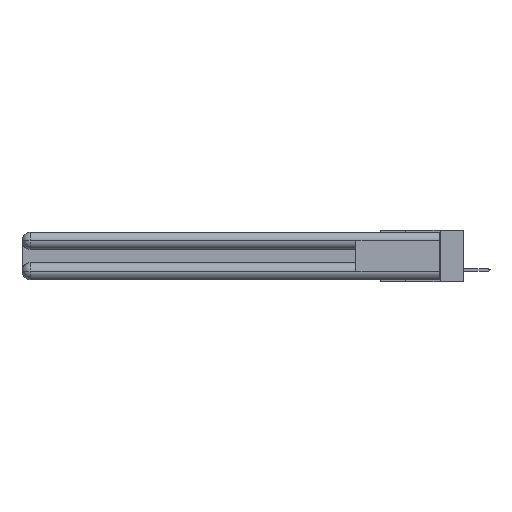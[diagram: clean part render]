
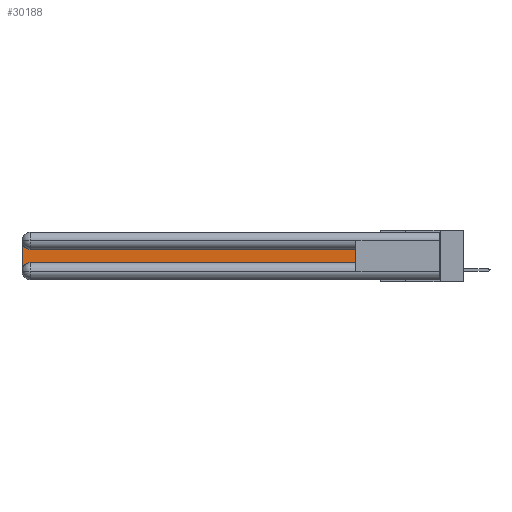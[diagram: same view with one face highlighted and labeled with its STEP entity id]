
A CAD part, left-side view. The second image highlights one B-rep face of the part: STEP entity #30188.
In plain terms, the highlighted planar face has unit normal (-1, 0, 0).
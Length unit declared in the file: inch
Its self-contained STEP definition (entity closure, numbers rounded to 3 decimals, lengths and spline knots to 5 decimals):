
#1519 = CIRCLE ( 'NONE', #22142, 0.06 ) ;
#1719 = CARTESIAN_POINT ( 'NONE',  ( 0.075, 3., -0.2175 ) ) ;
#1810 = LINE ( 'NONE', #1719, #28966 ) ;
#3148 = AXIS2_PLACEMENT_3D ( 'NONE', #26967, #32387, #3386 ) ;
#3265 = AXIS2_PLACEMENT_3D ( 'NONE', #26325, #26096, #31637 ) ;
#3386 = DIRECTION ( 'NONE',  ( 0., 0., -1. ) ) ;
#3557 = VECTOR ( 'NONE', #33413, 39.37008 ) ;
#4754 = ORIENTED_EDGE ( 'NONE', *, *, #8854, .T. ) ;
#5421 = CARTESIAN_POINT ( 'NONE',  ( 0.075, 0.6, -0.1225 ) ) ;
#5508 = VECTOR ( 'NONE', #16641, 39.37008 ) ;
#5574 = VERTEX_POINT ( 'NONE', #25280 ) ;
#8219 = VERTEX_POINT ( 'NONE', #13846 ) ;
#8854 = EDGE_CURVE ( 'NONE', #5574, #23633, #11387, .T. ) ;
#11274 = LINE ( 'NONE', #16530, #5508 ) ;
#11387 = CIRCLE ( 'NONE', #3148, 0.06 ) ;
#11801 = CARTESIAN_POINT ( 'NONE',  ( 0.075, 3., -0.2775 ) ) ;
#12319 = ORIENTED_EDGE ( 'NONE', *, *, #27634, .T. ) ;
#12581 = VERTEX_POINT ( 'NONE', #11801 ) ;
#13846 = CARTESIAN_POINT ( 'NONE',  ( 0.075, 2.94, -0.2175 ) ) ;
#13995 = ORIENTED_EDGE ( 'NONE', *, *, #14472, .T. ) ;
#14472 = EDGE_CURVE ( 'NONE', #23633, #12581, #1810, .T. ) ;
#16456 = CARTESIAN_POINT ( 'NONE',  ( 0.075, 2.94, -0.2775 ) ) ;
#16530 = CARTESIAN_POINT ( 'NONE',  ( 0.075, 0.6, -0.2175 ) ) ;
#16641 = DIRECTION ( 'NONE',  ( 0., -1., 0. ) ) ;
#18479 = EDGE_CURVE ( 'NONE', #8219, #20541, #11274, .T. ) ;
#20536 = CARTESIAN_POINT ( 'NONE',  ( 0.075, 0.6, -0.2175 ) ) ;
#20541 = VERTEX_POINT ( 'NONE', #26235 ) ;
#20821 = PLANE ( 'NONE',  #3265 ) ;
#21967 = EDGE_CURVE ( 'NONE', #12581, #8219, #1519, .T. ) ;
#22107 = FACE_OUTER_BOUND ( 'NONE', #31249, .T. ) ;
#22142 = AXIS2_PLACEMENT_3D ( 'NONE', #16456, #26698, #31997 ) ;
#22172 = VECTOR ( 'NONE', #33211, 39.37008 ) ;
#22885 = DIRECTION ( 'NONE',  ( 0., 0., -1. ) ) ;
#23083 = VERTEX_POINT ( 'NONE', #5421 ) ;
#23546 = CARTESIAN_POINT ( 'NONE',  ( 0.075, 3., -0.0625 ) ) ;
#23633 = VERTEX_POINT ( 'NONE', #23546 ) ;
#25280 = CARTESIAN_POINT ( 'NONE',  ( 0.075, 2.94, -0.1225 ) ) ;
#25559 = ORIENTED_EDGE ( 'NONE', *, *, #21967, .T. ) ;
#26096 = DIRECTION ( 'NONE',  ( 1., 0., 0. ) ) ;
#26235 = CARTESIAN_POINT ( 'NONE',  ( 0.075, 0.6, -0.2175 ) ) ;
#26325 = CARTESIAN_POINT ( 'NONE',  ( 0.075, 3., -0.1225 ) ) ;
#26698 = DIRECTION ( 'NONE',  ( 1., 0., 0. ) ) ;
#26967 = CARTESIAN_POINT ( 'NONE',  ( 0.075, 2.94, -0.0625 ) ) ;
#27580 = CARTESIAN_POINT ( 'NONE',  ( 0.075, 0.6, -0.1225 ) ) ;
#27634 = EDGE_CURVE ( 'NONE', #20541, #23083, #28610, .T. ) ;
#28610 = LINE ( 'NONE', #20536, #3557 ) ;
#28713 = LINE ( 'NONE', #27580, #22172 ) ;
#28966 = VECTOR ( 'NONE', #22885, 39.37008 ) ;
#29650 = EDGE_CURVE ( 'NONE', #23083, #5574, #28713, .T. ) ;
#30188 = ADVANCED_FACE ( 'NONE', ( #22107 ), #20821, .F. ) ;
#31249 = EDGE_LOOP ( 'NONE', ( #31764, #4754, #13995, #25559, #31790, #12319 ) ) ;
#31637 = DIRECTION ( 'NONE',  ( 0., 0., -1. ) ) ;
#31764 = ORIENTED_EDGE ( 'NONE', *, *, #29650, .T. ) ;
#31790 = ORIENTED_EDGE ( 'NONE', *, *, #18479, .T. ) ;
#31997 = DIRECTION ( 'NONE',  ( 0., 0., -1. ) ) ;
#32387 = DIRECTION ( 'NONE',  ( 1., 0., 0. ) ) ;
#33211 = DIRECTION ( 'NONE',  ( 0., 1., 0. ) ) ;
#33413 = DIRECTION ( 'NONE',  ( 0., 0., 1. ) ) ;
